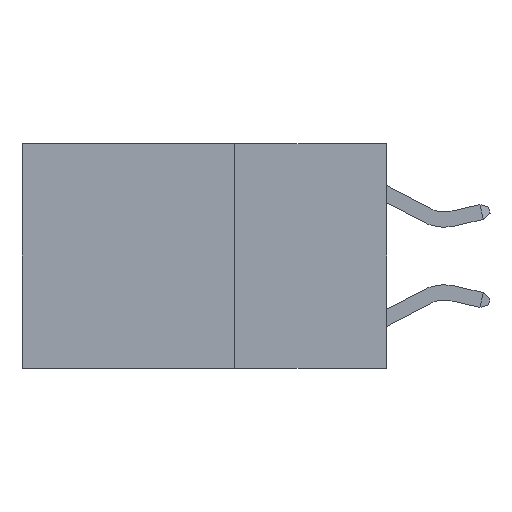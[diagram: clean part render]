
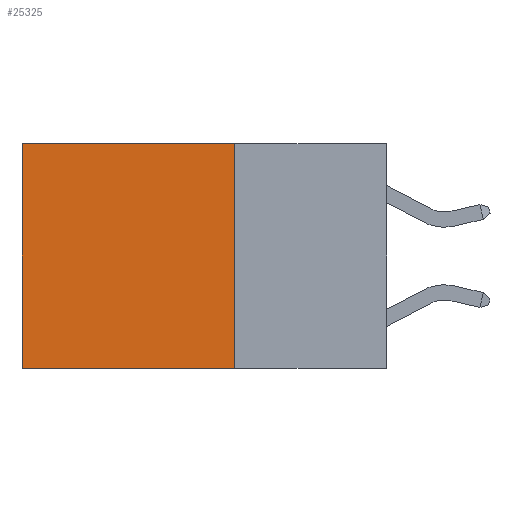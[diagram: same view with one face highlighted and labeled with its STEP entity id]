
A CAD part, left-side view. The second image highlights one B-rep face of the part: STEP entity #25325.
In plain terms, the highlighted planar face has unit normal (-1, 0, 0).
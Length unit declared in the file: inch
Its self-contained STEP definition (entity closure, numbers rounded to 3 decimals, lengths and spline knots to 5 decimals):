
#400 = EDGE_CURVE ( 'NONE', #30873, #7932, #15328, .T. ) ;
#2340 = LINE ( 'NONE', #29532, #10632 ) ;
#2669 = VECTOR ( 'NONE', #26354, 39.37008 ) ;
#4804 = ORIENTED_EDGE ( 'NONE', *, *, #400, .T. ) ;
#6083 = DIRECTION ( 'NONE',  ( 0., 0., -1. ) ) ;
#7932 = VERTEX_POINT ( 'NONE', #10831 ) ;
#8022 = FACE_OUTER_BOUND ( 'NONE', #27386, .T. ) ;
#8391 = CARTESIAN_POINT ( 'NONE',  ( 0.2625, 0.25, 0. ) ) ;
#8847 = ORIENTED_EDGE ( 'NONE', *, *, #23476, .F. ) ;
#9931 = EDGE_CURVE ( 'NONE', #25214, #24500, #15444, .T. ) ;
#10632 = VECTOR ( 'NONE', #12194, 39.37008 ) ;
#10831 = CARTESIAN_POINT ( 'NONE',  ( 0.2625, 0.6, -0.37 ) ) ;
#12194 = DIRECTION ( 'NONE',  ( 0., 1., 0. ) ) ;
#13322 = VECTOR ( 'NONE', #21268, 39.37008 ) ;
#15328 = LINE ( 'NONE', #25217, #19965 ) ;
#15444 = LINE ( 'NONE', #23710, #13322 ) ;
#15717 = ORIENTED_EDGE ( 'NONE', *, *, #9931, .F. ) ;
#16460 = LINE ( 'NONE', #8391, #2669 ) ;
#18200 = CARTESIAN_POINT ( 'NONE',  ( 0.2625, 0.25, 0. ) ) ;
#18358 = PLANE ( 'NONE',  #20633 ) ;
#19965 = VECTOR ( 'NONE', #23114, 39.37008 ) ;
#20633 = AXIS2_PLACEMENT_3D ( 'NONE', #27770, #28248, #6083 ) ;
#21268 = DIRECTION ( 'NONE',  ( 0., 0., -1. ) ) ;
#22836 = CARTESIAN_POINT ( 'NONE',  ( 0.2625, 0.6, 0. ) ) ;
#23114 = DIRECTION ( 'NONE',  ( 0., 0., -1. ) ) ;
#23476 = EDGE_CURVE ( 'NONE', #24500, #7932, #2340, .T. ) ;
#23710 = CARTESIAN_POINT ( 'NONE',  ( 0.2625, 0.25, 0. ) ) ;
#24500 = VERTEX_POINT ( 'NONE', #30385 ) ;
#25214 = VERTEX_POINT ( 'NONE', #18200 ) ;
#25217 = CARTESIAN_POINT ( 'NONE',  ( 0.2625, 0.6, 0. ) ) ;
#25325 = ADVANCED_FACE ( 'NONE', ( #8022 ), #18358, .F. ) ;
#26354 = DIRECTION ( 'NONE',  ( 0., 1., 0. ) ) ;
#27386 = EDGE_LOOP ( 'NONE', ( #4804, #8847, #15717, #31467 ) ) ;
#27770 = CARTESIAN_POINT ( 'NONE',  ( 0.2625, 0.25, 0. ) ) ;
#28248 = DIRECTION ( 'NONE',  ( 1., 0., 0. ) ) ;
#28323 = EDGE_CURVE ( 'NONE', #25214, #30873, #16460, .T. ) ;
#29532 = CARTESIAN_POINT ( 'NONE',  ( 0.2625, 0.25, -0.37 ) ) ;
#30385 = CARTESIAN_POINT ( 'NONE',  ( 0.2625, 0.25, -0.37 ) ) ;
#30873 = VERTEX_POINT ( 'NONE', #22836 ) ;
#31467 = ORIENTED_EDGE ( 'NONE', *, *, #28323, .T. ) ;
